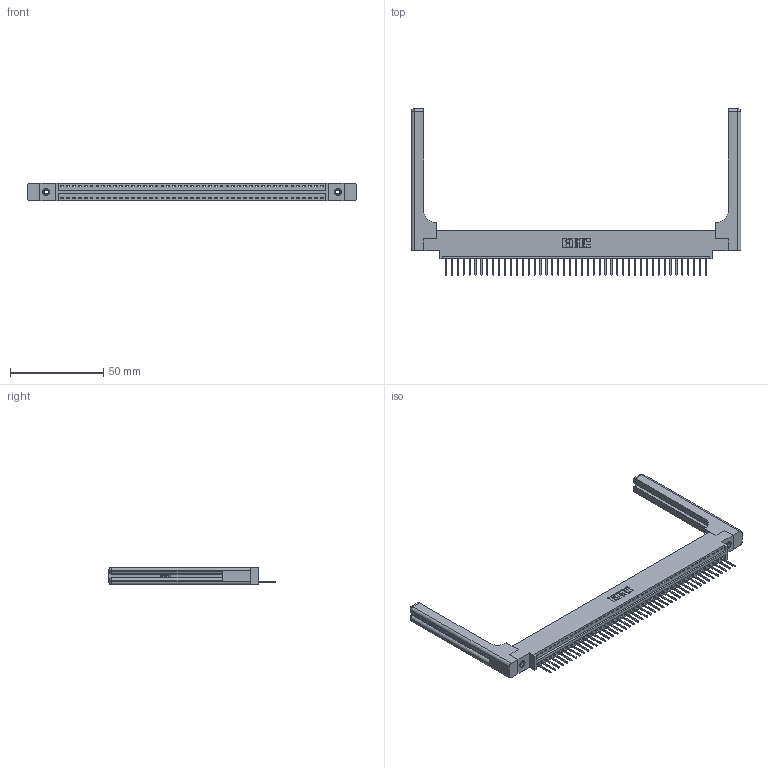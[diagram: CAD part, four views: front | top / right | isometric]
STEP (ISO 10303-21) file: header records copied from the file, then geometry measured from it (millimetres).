
FILE_DESCRIPTION (( 'STEP AP203' ), '1' );
FILE_NAME ('396-045-526-658.STEP', '2019-10-28T02:47:12', ( '' ), ( '' ), 'SwSTEP 2.0', 'SolidWorks 2016', '' );
FILE_SCHEMA (( 'CONFIG_CONTROL_DESIGN' ));
Length unit declared in the file: inch
Products named in the file (5): 346 Part_0.170 Offset - 0.156 Dia-TH; 396-045-526-658; 345-292-001_345-293-126; 345-250-001_345-250-001-102; 346-220-058_345-220-058
Assembly tree (50 placements, depth 2):
  396-045-526-658
    346 Part_0.170 Offset - 0.156 Dia-TH
    345-292-001_345-293-126  x45
    345-250-001_345-250-001-102  x2
    346-220-058_345-220-058  x2
Bounding box: 176.94 x 89.41 x 9.4 mm (x, y, z)
Volume: 24285.3 mm3; surface area: 26274.9 mm2
Topology: 50 solids, 50 shells, 2992 faces, 8927 edges, 5870 vertices
Faces by surface type: plane 2028, cylinder 904, bspline 36, cone 12, sphere 8, torus 4
Entity records: 32856 total; most frequent: CARTESIAN_POINT 6612, ORIENTED_EDGE 5388, DIRECTION 4760, EDGE_CURVE 2694, VECTOR 2290, LINE 2290, VERTEX_POINT 1786, AXIS2_PLACEMENT_3D 1235
